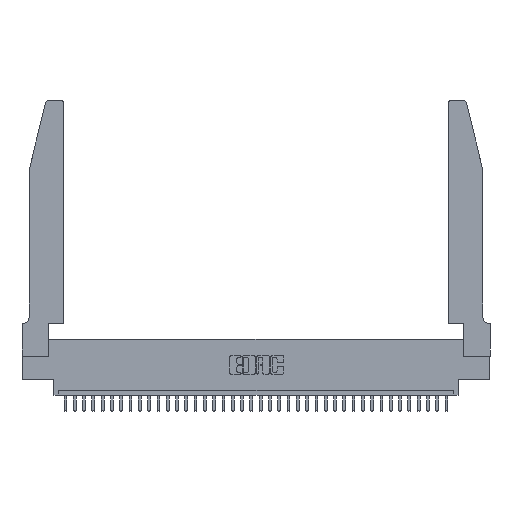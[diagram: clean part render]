
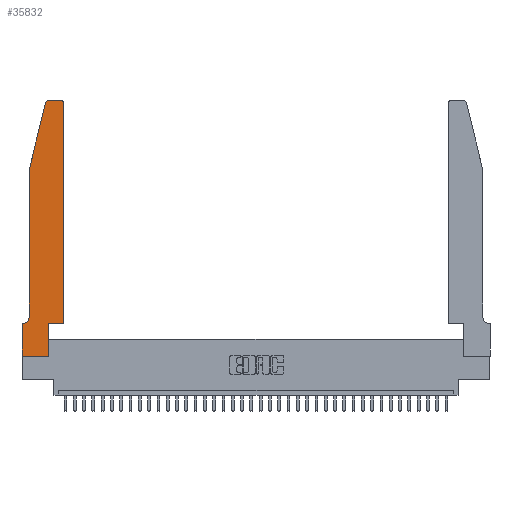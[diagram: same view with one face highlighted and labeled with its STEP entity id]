
A CAD part, top view. The second image highlights one B-rep face of the part: STEP entity #35832.
In plain terms, the highlighted planar face has unit normal (0, 0, 1).
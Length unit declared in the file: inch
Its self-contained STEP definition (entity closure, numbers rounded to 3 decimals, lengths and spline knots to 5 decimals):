
#110 = EDGE_CURVE ( 'NONE', #14971, #16541, #24944, .T. ) ;
#686 = EDGE_CURVE ( 'NONE', #15492, #33907, #16922, .T. ) ;
#1023 = CARTESIAN_POINT ( 'NONE',  ( 0., 0., 0.37 ) ) ;
#1370 = ORIENTED_EDGE ( 'NONE', *, *, #5525, .T. ) ;
#1379 = AXIS2_PLACEMENT_3D ( 'NONE', #4229, #29960, #7067 ) ;
#1455 = DIRECTION ( 'NONE',  ( -1., 0., 0. ) ) ;
#1979 = CARTESIAN_POINT ( 'NONE',  ( 0., 0., 0.37 ) ) ;
#2087 = DIRECTION ( 'NONE',  ( 0., 0., -1. ) ) ;
#2194 = CARTESIAN_POINT ( 'NONE',  ( 0.2605, 2.75, 0.37 ) ) ;
#2201 = VECTOR ( 'NONE', #18396, 39.37008 ) ;
#2305 = CARTESIAN_POINT ( 'NONE',  ( 0.0755, 2., 0.37 ) ) ;
#2605 = LINE ( 'NONE', #2194, #33153 ) ;
#2696 = DIRECTION ( 'NONE',  ( -1., 0., 0. ) ) ;
#2809 = ORIENTED_EDGE ( 'NONE', *, *, #12382, .T. ) ;
#2930 = EDGE_CURVE ( 'NONE', #3136, #20555, #22106, .T. ) ;
#3081 = DIRECTION ( 'NONE',  ( -0.239, -0.971, 0. ) ) ;
#3129 = ORIENTED_EDGE ( 'NONE', *, *, #21873, .T. ) ;
#3136 = VERTEX_POINT ( 'NONE', #7912 ) ;
#3280 = DIRECTION ( 'NONE',  ( 0., -1., 0. ) ) ;
#3499 = DIRECTION ( 'NONE',  ( 0., -1., 0. ) ) ;
#3524 = ORIENTED_EDGE ( 'NONE', *, *, #8495, .T. ) ;
#3659 = ORIENTED_EDGE ( 'NONE', *, *, #2930, .T. ) ;
#3691 = EDGE_CURVE ( 'NONE', #23263, #29172, #2605, .T. ) ;
#4151 = LINE ( 'NONE', #13912, #17407 ) ;
#4229 = CARTESIAN_POINT ( 'NONE',  ( 0., 0.35, 0.37 ) ) ;
#5525 = EDGE_CURVE ( 'NONE', #16541, #13227, #4151, .T. ) ;
#5737 = CARTESIAN_POINT ( 'NONE',  ( 0.4505, 0.35, 0.37 ) ) ;
#6711 = AXIS2_PLACEMENT_3D ( 'NONE', #30667, #2087, #2696 ) ;
#7067 = DIRECTION ( 'NONE',  ( 1., 0., 0. ) ) ;
#7912 = CARTESIAN_POINT ( 'NONE',  ( 0.0055, 0.35, 0.37 ) ) ;
#7921 = LINE ( 'NONE', #10418, #14122 ) ;
#8495 = EDGE_CURVE ( 'NONE', #33907, #34542, #14104, .T. ) ;
#8656 = EDGE_CURVE ( 'NONE', #13227, #3136, #28724, .T. ) ;
#9600 = DIRECTION ( 'NONE',  ( 0., 0., 1. ) ) ;
#9792 = CARTESIAN_POINT ( 'NONE',  ( 0., 0.35, 0.37 ) ) ;
#10418 = CARTESIAN_POINT ( 'NONE',  ( 0.4505, 0.35, 0.37 ) ) ;
#11641 = AXIS2_PLACEMENT_3D ( 'NONE', #26584, #9600, #12191 ) ;
#12191 = DIRECTION ( 'NONE',  ( 1., 0., 0. ) ) ;
#12382 = EDGE_CURVE ( 'NONE', #20555, #15492, #35398, .T. ) ;
#12863 = ORIENTED_EDGE ( 'NONE', *, *, #110, .T. ) ;
#13122 = CARTESIAN_POINT ( 'NONE',  ( 0.284, 2.75, 0.37 ) ) ;
#13227 = VERTEX_POINT ( 'NONE', #21920 ) ;
#13912 = CARTESIAN_POINT ( 'NONE',  ( 0.0755, 2., 0.37 ) ) ;
#14104 = LINE ( 'NONE', #23841, #2201 ) ;
#14122 = VECTOR ( 'NONE', #30376, 39.37008 ) ;
#14188 = CARTESIAN_POINT ( 'NONE',  ( 0.4505, 2.72, 0.37 ) ) ;
#14971 = VERTEX_POINT ( 'NONE', #19707 ) ;
#15492 = VERTEX_POINT ( 'NONE', #26807 ) ;
#15524 = CARTESIAN_POINT ( 'NONE',  ( 0.4205, 2.72, 0.37 ) ) ;
#16508 = LINE ( 'NONE', #29986, #18283 ) ;
#16541 = VERTEX_POINT ( 'NONE', #2305 ) ;
#16922 = LINE ( 'NONE', #1979, #26714 ) ;
#17105 = ORIENTED_EDGE ( 'NONE', *, *, #3691, .T. ) ;
#17407 = VECTOR ( 'NONE', #3280, 39.37008 ) ;
#17423 = VECTOR ( 'NONE', #3081, 39.37008 ) ;
#18283 = VECTOR ( 'NONE', #26780, 39.37008 ) ;
#18380 = DIRECTION ( 'NONE',  ( 0., 0., 1. ) ) ;
#18396 = DIRECTION ( 'NONE',  ( 0., 1., 0. ) ) ;
#19160 = EDGE_CURVE ( 'NONE', #31122, #23263, #19596, .T. ) ;
#19596 = CIRCLE ( 'NONE', #33707, 0.03 ) ;
#19707 = CARTESIAN_POINT ( 'NONE',  ( 0.25487, 2.72718, 0.37 ) ) ;
#20042 = ORIENTED_EDGE ( 'NONE', *, *, #8656, .T. ) ;
#20555 = VERTEX_POINT ( 'NONE', #9792 ) ;
#21496 = DIRECTION ( 'NONE',  ( 1., 0., 0. ) ) ;
#21583 = DIRECTION ( 'NONE',  ( -1., 0., 0. ) ) ;
#21873 = EDGE_CURVE ( 'NONE', #34960, #31122, #7921, .T. ) ;
#21920 = CARTESIAN_POINT ( 'NONE',  ( 0.0755, 0.42, 0.37 ) ) ;
#22106 = LINE ( 'NONE', #35705, #29659 ) ;
#22164 = EDGE_LOOP ( 'NONE', ( #17105, #31727, #12863, #1370, #20042, #3659, #2809, #31261, #3524, #26028, #3129, #26327 ) ) ;
#23263 = VERTEX_POINT ( 'NONE', #31521 ) ;
#23841 = CARTESIAN_POINT ( 'NONE',  ( 0.2865, 0.35, 0.37 ) ) ;
#24944 = LINE ( 'NONE', #34140, #17423 ) ;
#26028 = ORIENTED_EDGE ( 'NONE', *, *, #35213, .T. ) ;
#26074 = CARTESIAN_POINT ( 'NONE',  ( 0.2865, 0., 0.37 ) ) ;
#26327 = ORIENTED_EDGE ( 'NONE', *, *, #19160, .T. ) ;
#26584 = CARTESIAN_POINT ( 'NONE',  ( 0.284, 2.72, 0.37 ) ) ;
#26714 = VECTOR ( 'NONE', #21496, 39.37008 ) ;
#26780 = DIRECTION ( 'NONE',  ( 1., 0., 0. ) ) ;
#26807 = CARTESIAN_POINT ( 'NONE',  ( 0., 0., 0.37 ) ) ;
#28724 = CIRCLE ( 'NONE', #6711, 0.07 ) ;
#29172 = VERTEX_POINT ( 'NONE', #13122 ) ;
#29659 = VECTOR ( 'NONE', #1455, 39.37008 ) ;
#29718 = PLANE ( 'NONE',  #1379 ) ;
#29774 = FACE_OUTER_BOUND ( 'NONE', #22164, .T. ) ;
#29960 = DIRECTION ( 'NONE',  ( 0., 0., 1. ) ) ;
#29986 = CARTESIAN_POINT ( 'NONE',  ( 0.4505, 0.35, 0.37 ) ) ;
#30376 = DIRECTION ( 'NONE',  ( 0., 1., 0. ) ) ;
#30667 = CARTESIAN_POINT ( 'NONE',  ( 0.0055, 0.42, 0.37 ) ) ;
#30978 = VECTOR ( 'NONE', #3499, 39.37008 ) ;
#31122 = VERTEX_POINT ( 'NONE', #14188 ) ;
#31261 = ORIENTED_EDGE ( 'NONE', *, *, #686, .T. ) ;
#31521 = CARTESIAN_POINT ( 'NONE',  ( 0.4205, 2.75, 0.37 ) ) ;
#31727 = ORIENTED_EDGE ( 'NONE', *, *, #32094, .T. ) ;
#32094 = EDGE_CURVE ( 'NONE', #29172, #14971, #33144, .T. ) ;
#33144 = CIRCLE ( 'NONE', #11641, 0.03 ) ;
#33153 = VECTOR ( 'NONE', #21583, 39.37008 ) ;
#33707 = AXIS2_PLACEMENT_3D ( 'NONE', #15524, #18380, #35085 ) ;
#33907 = VERTEX_POINT ( 'NONE', #26074 ) ;
#34140 = CARTESIAN_POINT ( 'NONE',  ( 0.0755, 2., 0.37 ) ) ;
#34542 = VERTEX_POINT ( 'NONE', #35200 ) ;
#34960 = VERTEX_POINT ( 'NONE', #5737 ) ;
#35085 = DIRECTION ( 'NONE',  ( 1., 0., 0. ) ) ;
#35200 = CARTESIAN_POINT ( 'NONE',  ( 0.2865, 0.35, 0.37 ) ) ;
#35213 = EDGE_CURVE ( 'NONE', #34542, #34960, #16508, .T. ) ;
#35398 = LINE ( 'NONE', #1023, #30978 ) ;
#35705 = CARTESIAN_POINT ( 'NONE',  ( 0.0755, 0.35, 0.37 ) ) ;
#35832 = ADVANCED_FACE ( 'NONE', ( #29774 ), #29718, .T. ) ;
